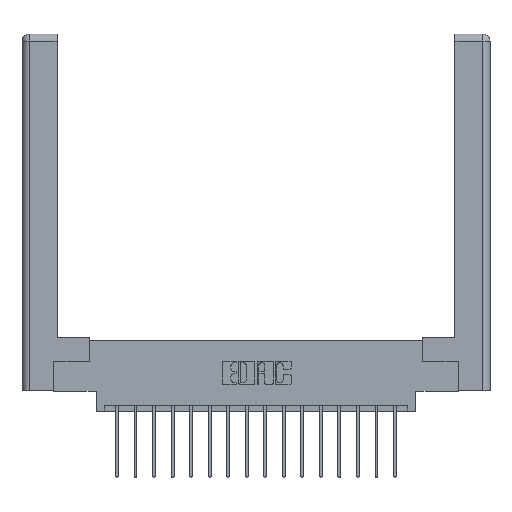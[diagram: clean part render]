
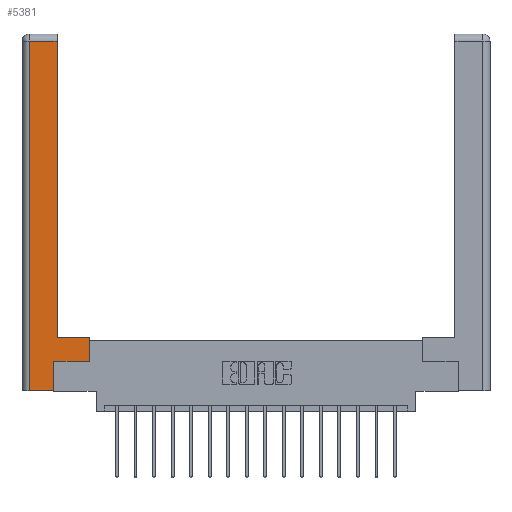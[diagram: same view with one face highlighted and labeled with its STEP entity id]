
A CAD part, top view. The second image highlights one B-rep face of the part: STEP entity #5381.
In plain terms, the highlighted planar face has unit normal (0, 0, 1).
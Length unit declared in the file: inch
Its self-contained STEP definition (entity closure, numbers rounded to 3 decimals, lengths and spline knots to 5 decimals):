
#187 = CARTESIAN_POINT ( 'NONE',  ( 0.295, 0.45, 0. ) ) ;
#352 = ORIENTED_EDGE ( 'NONE', *, *, #2604, .T. ) ;
#561 = VERTEX_POINT ( 'NONE', #11959 ) ;
#923 = CARTESIAN_POINT ( 'NONE',  ( 0.295, 3., 0. ) ) ;
#1097 = LINE ( 'NONE', #13813, #4675 ) ;
#1284 = VECTOR ( 'NONE', #17222, 39.37008 ) ;
#1798 = EDGE_CURVE ( 'NONE', #13899, #2208, #7363, .T. ) ;
#1849 = EDGE_CURVE ( 'NONE', #16976, #561, #2663, .T. ) ;
#2067 = VERTEX_POINT ( 'NONE', #10858 ) ;
#2208 = VERTEX_POINT ( 'NONE', #7419 ) ;
#2468 = VECTOR ( 'NONE', #10955, 39.37008 ) ;
#2604 = EDGE_CURVE ( 'NONE', #2208, #2067, #16048, .T. ) ;
#2663 = LINE ( 'NONE', #187, #17228 ) ;
#3386 = EDGE_CURVE ( 'NONE', #2067, #9117, #11541, .T. ) ;
#3575 = EDGE_CURVE ( 'NONE', #8929, #16976, #7308, .T. ) ;
#3737 = ORIENTED_EDGE ( 'NONE', *, *, #1798, .T. ) ;
#3991 = PLANE ( 'NONE',  #17294 ) ;
#4675 = VECTOR ( 'NONE', #15259, 39.37008 ) ;
#5381 = ADVANCED_FACE ( 'NONE', ( #11808 ), #3991, .F. ) ;
#5721 = CARTESIAN_POINT ( 'NONE',  ( 0.565, 0.245, 0. ) ) ;
#6924 = ORIENTED_EDGE ( 'NONE', *, *, #1849, .T. ) ;
#7023 = CARTESIAN_POINT ( 'NONE',  ( 0., 0., 0. ) ) ;
#7308 = LINE ( 'NONE', #7375, #11520 ) ;
#7363 = LINE ( 'NONE', #11027, #14047 ) ;
#7375 = CARTESIAN_POINT ( 'NONE',  ( 0.565, 0.45, 0. ) ) ;
#7419 = CARTESIAN_POINT ( 'NONE',  ( 0.0615, 2.94, 0. ) ) ;
#7536 = VECTOR ( 'NONE', #14293, 39.37008 ) ;
#7741 = ORIENTED_EDGE ( 'NONE', *, *, #17185, .T. ) ;
#8197 = CARTESIAN_POINT ( 'NONE',  ( 0.0615, 0., 0. ) ) ;
#8663 = CARTESIAN_POINT ( 'NONE',  ( 0.565, 0.45, 0. ) ) ;
#8830 = EDGE_LOOP ( 'NONE', ( #7741, #3737, #352, #12090, #10754, #11887, #16261, #6924 ) ) ;
#8929 = VERTEX_POINT ( 'NONE', #5721 ) ;
#9117 = VERTEX_POINT ( 'NONE', #9715 ) ;
#9224 = EDGE_CURVE ( 'NONE', #15268, #8929, #13943, .T. ) ;
#9715 = CARTESIAN_POINT ( 'NONE',  ( 0.265, 0., 0. ) ) ;
#10162 = DIRECTION ( 'NONE',  ( -1., 0., 0. ) ) ;
#10754 = ORIENTED_EDGE ( 'NONE', *, *, #12147, .T. ) ;
#10858 = CARTESIAN_POINT ( 'NONE',  ( 0.0615, 0., 0. ) ) ;
#10955 = DIRECTION ( 'NONE',  ( 0., 1., 0. ) ) ;
#11014 = DIRECTION ( 'NONE',  ( 0., 0., -1. ) ) ;
#11027 = CARTESIAN_POINT ( 'NONE',  ( 0.0615, 2.94, 0. ) ) ;
#11520 = VECTOR ( 'NONE', #15997, 39.37008 ) ;
#11541 = LINE ( 'NONE', #12782, #1284 ) ;
#11808 = FACE_OUTER_BOUND ( 'NONE', #8830, .T. ) ;
#11887 = ORIENTED_EDGE ( 'NONE', *, *, #9224, .T. ) ;
#11959 = CARTESIAN_POINT ( 'NONE',  ( 0.295, 0.45, 0. ) ) ;
#12090 = ORIENTED_EDGE ( 'NONE', *, *, #3386, .T. ) ;
#12147 = EDGE_CURVE ( 'NONE', #9117, #15268, #1097, .T. ) ;
#12503 = CARTESIAN_POINT ( 'NONE',  ( 0.265, 0.245, 0. ) ) ;
#12782 = CARTESIAN_POINT ( 'NONE',  ( 0.265, 0., 0. ) ) ;
#12937 = CARTESIAN_POINT ( 'NONE',  ( 0.565, 0.245, 0. ) ) ;
#13813 = CARTESIAN_POINT ( 'NONE',  ( 0.265, 0.245, 0. ) ) ;
#13899 = VERTEX_POINT ( 'NONE', #14005 ) ;
#13943 = LINE ( 'NONE', #12937, #14397 ) ;
#14005 = CARTESIAN_POINT ( 'NONE',  ( 0.295, 2.94, 0. ) ) ;
#14047 = VECTOR ( 'NONE', #15394, 39.37008 ) ;
#14293 = DIRECTION ( 'NONE',  ( 0., -1., 0. ) ) ;
#14397 = VECTOR ( 'NONE', #14458, 39.37008 ) ;
#14458 = DIRECTION ( 'NONE',  ( 1., 0., 0. ) ) ;
#15259 = DIRECTION ( 'NONE',  ( 0., 1., 0. ) ) ;
#15268 = VERTEX_POINT ( 'NONE', #12503 ) ;
#15394 = DIRECTION ( 'NONE',  ( -1., 0., 0. ) ) ;
#15997 = DIRECTION ( 'NONE',  ( 0., 1., 0. ) ) ;
#16048 = LINE ( 'NONE', #8197, #7536 ) ;
#16261 = ORIENTED_EDGE ( 'NONE', *, *, #3575, .T. ) ;
#16976 = VERTEX_POINT ( 'NONE', #8663 ) ;
#17185 = EDGE_CURVE ( 'NONE', #561, #13899, #17715, .T. ) ;
#17222 = DIRECTION ( 'NONE',  ( 1., 0., 0. ) ) ;
#17228 = VECTOR ( 'NONE', #10162, 39.37008 ) ;
#17294 = AXIS2_PLACEMENT_3D ( 'NONE', #7023, #11014, #18424 ) ;
#17715 = LINE ( 'NONE', #923, #2468 ) ;
#18424 = DIRECTION ( 'NONE',  ( -1., 0., 0. ) ) ;
